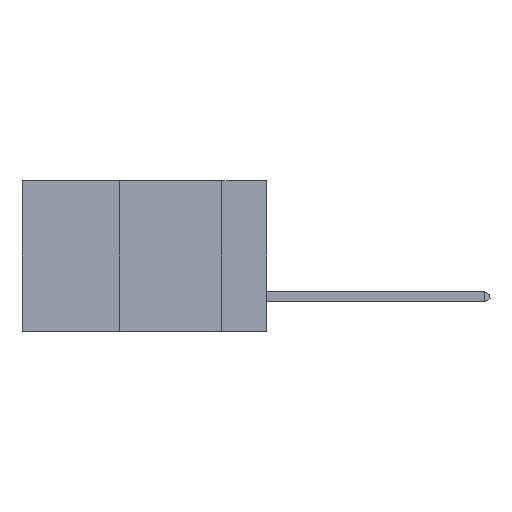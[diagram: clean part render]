
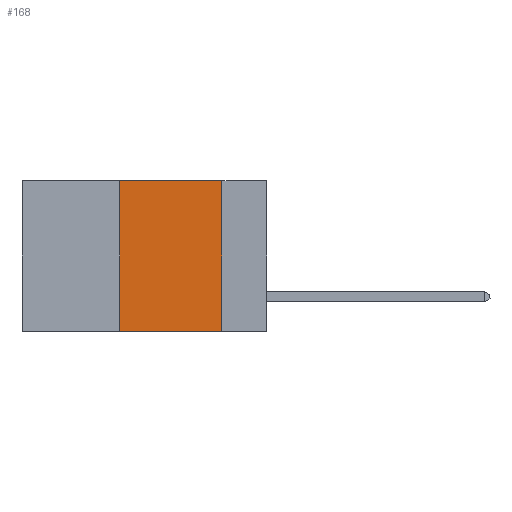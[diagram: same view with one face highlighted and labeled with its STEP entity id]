
A CAD part, left-side view. The second image highlights one B-rep face of the part: STEP entity #168.
In plain terms, the highlighted planar face has unit normal (-1, 0, 0).
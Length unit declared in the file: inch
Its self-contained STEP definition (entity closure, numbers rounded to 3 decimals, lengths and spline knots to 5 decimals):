
#168 = ADVANCED_FACE ( 'NONE', ( #1159 ), #5801, .F. ) ;
#813 = ORIENTED_EDGE ( 'NONE', *, *, #7491, .F. ) ;
#924 = CARTESIAN_POINT ( 'NONE',  ( 0., 0.11, 0. ) ) ;
#1159 = FACE_OUTER_BOUND ( 'NONE', #7954, .T. ) ;
#1719 = CARTESIAN_POINT ( 'NONE',  ( 0., 0.11, 0. ) ) ;
#2256 = VECTOR ( 'NONE', #4497, 39.37008 ) ;
#2520 = ORIENTED_EDGE ( 'NONE', *, *, #2838, .F. ) ;
#2838 = EDGE_CURVE ( 'NONE', #9189, #11233, #12311, .T. ) ;
#3026 = CARTESIAN_POINT ( 'NONE',  ( 0., 0.36, -0.37 ) ) ;
#3739 = AXIS2_PLACEMENT_3D ( 'NONE', #11478, #7177, #12169 ) ;
#3875 = LINE ( 'NONE', #1719, #6528 ) ;
#4497 = DIRECTION ( 'NONE',  ( 0., 0., 1. ) ) ;
#5007 = EDGE_CURVE ( 'NONE', #9189, #5145, #9635, .T. ) ;
#5145 = VERTEX_POINT ( 'NONE', #7281 ) ;
#5656 = ORIENTED_EDGE ( 'NONE', *, *, #5007, .T. ) ;
#5801 = PLANE ( 'NONE',  #3739 ) ;
#5840 = DIRECTION ( 'NONE',  ( 0., 0., -1. ) ) ;
#6528 = VECTOR ( 'NONE', #5840, 39.37008 ) ;
#6610 = CARTESIAN_POINT ( 'NONE',  ( 0., 0.36, 0. ) ) ;
#7132 = DIRECTION ( 'NONE',  ( 0., -1., 0. ) ) ;
#7177 = DIRECTION ( 'NONE',  ( 1., 0., 0. ) ) ;
#7281 = CARTESIAN_POINT ( 'NONE',  ( 0., 0.11, -0.37 ) ) ;
#7491 = EDGE_CURVE ( 'NONE', #11233, #10605, #10743, .T. ) ;
#7594 = VECTOR ( 'NONE', #10270, 39.37008 ) ;
#7954 = EDGE_LOOP ( 'NONE', ( #11556, #813, #2520, #5656 ) ) ;
#8828 = CARTESIAN_POINT ( 'NONE',  ( 0., 0.6, -0.37 ) ) ;
#9189 = VERTEX_POINT ( 'NONE', #3026 ) ;
#9635 = LINE ( 'NONE', #8828, #7594 ) ;
#10201 = CARTESIAN_POINT ( 'NONE',  ( 0., 0.36, 0. ) ) ;
#10270 = DIRECTION ( 'NONE',  ( 0., -1., 0. ) ) ;
#10420 = EDGE_CURVE ( 'NONE', #10605, #5145, #3875, .T. ) ;
#10605 = VERTEX_POINT ( 'NONE', #924 ) ;
#10743 = LINE ( 'NONE', #11782, #11040 ) ;
#11040 = VECTOR ( 'NONE', #7132, 39.37008 ) ;
#11233 = VERTEX_POINT ( 'NONE', #10201 ) ;
#11478 = CARTESIAN_POINT ( 'NONE',  ( 0., 0.6, 0. ) ) ;
#11556 = ORIENTED_EDGE ( 'NONE', *, *, #10420, .F. ) ;
#11782 = CARTESIAN_POINT ( 'NONE',  ( 0., 0.6, 0. ) ) ;
#12169 = DIRECTION ( 'NONE',  ( 0., 0., -1. ) ) ;
#12311 = LINE ( 'NONE', #6610, #2256 ) ;
